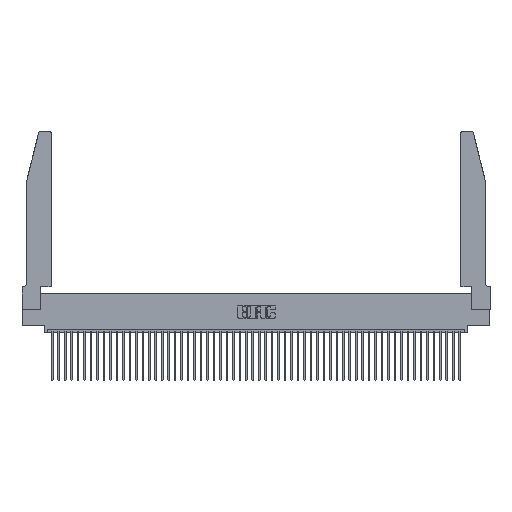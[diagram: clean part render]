
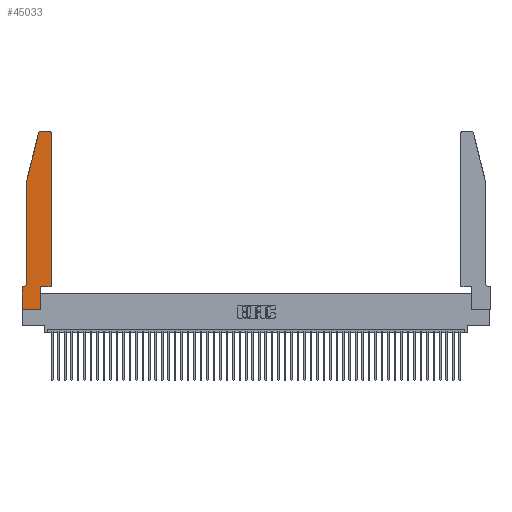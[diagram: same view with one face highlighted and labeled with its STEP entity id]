
A CAD part, top view. The second image highlights one B-rep face of the part: STEP entity #45033.
In plain terms, the highlighted planar face has unit normal (0, 0, 1).
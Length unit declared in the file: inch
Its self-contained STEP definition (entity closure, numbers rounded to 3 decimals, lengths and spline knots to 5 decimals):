
#310 = EDGE_CURVE ( 'NONE', #7079, #7900, #16074, .T. ) ;
#844 = DIRECTION ( 'NONE',  ( -0.239, -0.971, 0. ) ) ;
#1016 = CARTESIAN_POINT ( 'NONE',  ( 0.0755, 2., 0.37 ) ) ;
#1323 = DIRECTION ( 'NONE',  ( 0., 0., 1. ) ) ;
#1822 = VERTEX_POINT ( 'NONE', #5281 ) ;
#2116 = LINE ( 'NONE', #24383, #26653 ) ;
#2177 = DIRECTION ( 'NONE',  ( 1., 0., 0. ) ) ;
#2615 = EDGE_CURVE ( 'NONE', #30392, #1822, #43656, .T. ) ;
#2825 = DIRECTION ( 'NONE',  ( -1., 0., 0. ) ) ;
#3468 = EDGE_CURVE ( 'NONE', #40516, #39621, #15827, .T. ) ;
#3479 = CARTESIAN_POINT ( 'NONE',  ( 0., 0., 0.37 ) ) ;
#4533 = DIRECTION ( 'NONE',  ( 0., 0., -1. ) ) ;
#4553 = EDGE_CURVE ( 'NONE', #36430, #10673, #25166, .T. ) ;
#5281 = CARTESIAN_POINT ( 'NONE',  ( 0.0055, 0.35, 0.37 ) ) ;
#5951 = VECTOR ( 'NONE', #11165, 39.37008 ) ;
#6889 = VERTEX_POINT ( 'NONE', #39314 ) ;
#7079 = VERTEX_POINT ( 'NONE', #12042 ) ;
#7628 = LINE ( 'NONE', #10386, #35330 ) ;
#7900 = VERTEX_POINT ( 'NONE', #20980 ) ;
#7938 = ORIENTED_EDGE ( 'NONE', *, *, #14414, .T. ) ;
#9127 = DIRECTION ( 'NONE',  ( -1., 0., 0. ) ) ;
#9641 = FACE_OUTER_BOUND ( 'NONE', #26294, .T. ) ;
#9767 = CARTESIAN_POINT ( 'NONE',  ( 0.4505, 0.35, 0.37 ) ) ;
#10136 = CARTESIAN_POINT ( 'NONE',  ( 0.2865, 0.35, 0.37 ) ) ;
#10386 = CARTESIAN_POINT ( 'NONE',  ( 0.4505, 0.35, 0.37 ) ) ;
#10673 = VERTEX_POINT ( 'NONE', #15506 ) ;
#10934 = DIRECTION ( 'NONE',  ( 1., 0., 0. ) ) ;
#11165 = DIRECTION ( 'NONE',  ( 0., 1., 0. ) ) ;
#11215 = LINE ( 'NONE', #16075, #40210 ) ;
#11860 = ORIENTED_EDGE ( 'NONE', *, *, #44068, .T. ) ;
#12023 = VERTEX_POINT ( 'NONE', #12801 ) ;
#12042 = CARTESIAN_POINT ( 'NONE',  ( 0., 0.35, 0.37 ) ) ;
#12210 = VECTOR ( 'NONE', #10934, 39.37008 ) ;
#12801 = CARTESIAN_POINT ( 'NONE',  ( 0.4505, 2.72, 0.37 ) ) ;
#12820 = EDGE_CURVE ( 'NONE', #7900, #18543, #29220, .T. ) ;
#14414 = EDGE_CURVE ( 'NONE', #6889, #36430, #41603, .T. ) ;
#14743 = LINE ( 'NONE', #51143, #5951 ) ;
#15317 = CARTESIAN_POINT ( 'NONE',  ( 0.0755, 0.42, 0.37 ) ) ;
#15506 = CARTESIAN_POINT ( 'NONE',  ( 0.0755, 2., 0.37 ) ) ;
#15827 = LINE ( 'NONE', #9767, #46699 ) ;
#16074 = LINE ( 'NONE', #3479, #35579 ) ;
#16075 = CARTESIAN_POINT ( 'NONE',  ( 0.0755, 0.35, 0.37 ) ) ;
#16235 = DIRECTION ( 'NONE',  ( -1., 0., 0. ) ) ;
#16953 = ORIENTED_EDGE ( 'NONE', *, *, #310, .T. ) ;
#16961 = VECTOR ( 'NONE', #844, 39.37008 ) ;
#17180 = CARTESIAN_POINT ( 'NONE',  ( 0., 0.35, 0.37 ) ) ;
#18543 = VERTEX_POINT ( 'NONE', #35115 ) ;
#18546 = CARTESIAN_POINT ( 'NONE',  ( 0., 0., 0.37 ) ) ;
#18878 = CARTESIAN_POINT ( 'NONE',  ( 0.4205, 2.75, 0.37 ) ) ;
#20162 = ORIENTED_EDGE ( 'NONE', *, *, #22331, .T. ) ;
#20730 = EDGE_CURVE ( 'NONE', #39621, #12023, #7628, .T. ) ;
#20980 = CARTESIAN_POINT ( 'NONE',  ( 0., 0., 0.37 ) ) ;
#21754 = CARTESIAN_POINT ( 'NONE',  ( 0.284, 2.72, 0.37 ) ) ;
#22331 = EDGE_CURVE ( 'NONE', #1822, #7079, #11215, .T. ) ;
#22480 = EDGE_CURVE ( 'NONE', #12023, #38680, #33842, .T. ) ;
#22947 = CARTESIAN_POINT ( 'NONE',  ( 0.2605, 2.75, 0.37 ) ) ;
#23137 = ORIENTED_EDGE ( 'NONE', *, *, #44459, .T. ) ;
#23261 = DIRECTION ( 'NONE',  ( 0., 1., 0. ) ) ;
#23520 = ORIENTED_EDGE ( 'NONE', *, *, #2615, .T. ) ;
#23722 = AXIS2_PLACEMENT_3D ( 'NONE', #25337, #4533, #9127 ) ;
#24383 = CARTESIAN_POINT ( 'NONE',  ( 0.0755, 2., 0.37 ) ) ;
#24700 = AXIS2_PLACEMENT_3D ( 'NONE', #21754, #29823, #2177 ) ;
#25120 = PLANE ( 'NONE',  #40630 ) ;
#25166 = LINE ( 'NONE', #1016, #16961 ) ;
#25337 = CARTESIAN_POINT ( 'NONE',  ( 0.0055, 0.42, 0.37 ) ) ;
#25743 = DIRECTION ( 'NONE',  ( 0., -1., 0. ) ) ;
#25884 = CARTESIAN_POINT ( 'NONE',  ( 0.4205, 2.72, 0.37 ) ) ;
#26294 = EDGE_LOOP ( 'NONE', ( #38445, #7938, #37822, #23137, #23520, #20162, #16953, #37099, #11860, #48794, #29044, #31838 ) ) ;
#26484 = LINE ( 'NONE', #22947, #35921 ) ;
#26653 = VECTOR ( 'NONE', #25743, 39.37008 ) ;
#29044 = ORIENTED_EDGE ( 'NONE', *, *, #20730, .T. ) ;
#29220 = LINE ( 'NONE', #18546, #12210 ) ;
#29270 = CARTESIAN_POINT ( 'NONE',  ( 0.25487, 2.72718, 0.37 ) ) ;
#29823 = DIRECTION ( 'NONE',  ( 0., 0., 1. ) ) ;
#30392 = VERTEX_POINT ( 'NONE', #15317 ) ;
#31838 = ORIENTED_EDGE ( 'NONE', *, *, #22480, .T. ) ;
#33842 = CIRCLE ( 'NONE', #50925, 0.03 ) ;
#35115 = CARTESIAN_POINT ( 'NONE',  ( 0.2865, 0., 0.37 ) ) ;
#35330 = VECTOR ( 'NONE', #23261, 39.37008 ) ;
#35579 = VECTOR ( 'NONE', #47711, 39.37008 ) ;
#35921 = VECTOR ( 'NONE', #2825, 39.37008 ) ;
#36430 = VERTEX_POINT ( 'NONE', #29270 ) ;
#37099 = ORIENTED_EDGE ( 'NONE', *, *, #12820, .T. ) ;
#37822 = ORIENTED_EDGE ( 'NONE', *, *, #4553, .T. ) ;
#38445 = ORIENTED_EDGE ( 'NONE', *, *, #38706, .T. ) ;
#38680 = VERTEX_POINT ( 'NONE', #18878 ) ;
#38706 = EDGE_CURVE ( 'NONE', #38680, #6889, #26484, .T. ) ;
#39314 = CARTESIAN_POINT ( 'NONE',  ( 0.284, 2.75, 0.37 ) ) ;
#39621 = VERTEX_POINT ( 'NONE', #43351 ) ;
#40210 = VECTOR ( 'NONE', #16235, 39.37008 ) ;
#40516 = VERTEX_POINT ( 'NONE', #10136 ) ;
#40630 = AXIS2_PLACEMENT_3D ( 'NONE', #17180, #1323, #41994 ) ;
#41546 = DIRECTION ( 'NONE',  ( 0., 0., 1. ) ) ;
#41603 = CIRCLE ( 'NONE', #24700, 0.03 ) ;
#41994 = DIRECTION ( 'NONE',  ( 1., 0., 0. ) ) ;
#43351 = CARTESIAN_POINT ( 'NONE',  ( 0.4505, 0.35, 0.37 ) ) ;
#43656 = CIRCLE ( 'NONE', #23722, 0.07 ) ;
#44068 = EDGE_CURVE ( 'NONE', #18543, #40516, #14743, .T. ) ;
#44459 = EDGE_CURVE ( 'NONE', #10673, #30392, #2116, .T. ) ;
#45033 = ADVANCED_FACE ( 'NONE', ( #9641 ), #25120, .T. ) ;
#46406 = DIRECTION ( 'NONE',  ( 1., 0., 0. ) ) ;
#46699 = VECTOR ( 'NONE', #46406, 39.37008 ) ;
#47711 = DIRECTION ( 'NONE',  ( 0., -1., 0. ) ) ;
#48794 = ORIENTED_EDGE ( 'NONE', *, *, #3468, .T. ) ;
#49845 = DIRECTION ( 'NONE',  ( 1., 0., 0. ) ) ;
#50925 = AXIS2_PLACEMENT_3D ( 'NONE', #25884, #41546, #49845 ) ;
#51143 = CARTESIAN_POINT ( 'NONE',  ( 0.2865, 0.35, 0.37 ) ) ;
